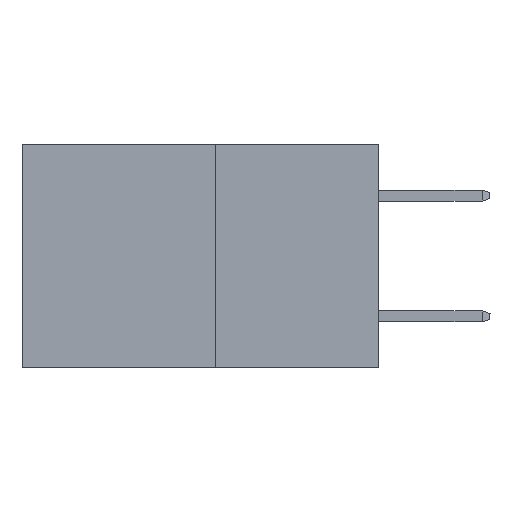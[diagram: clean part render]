
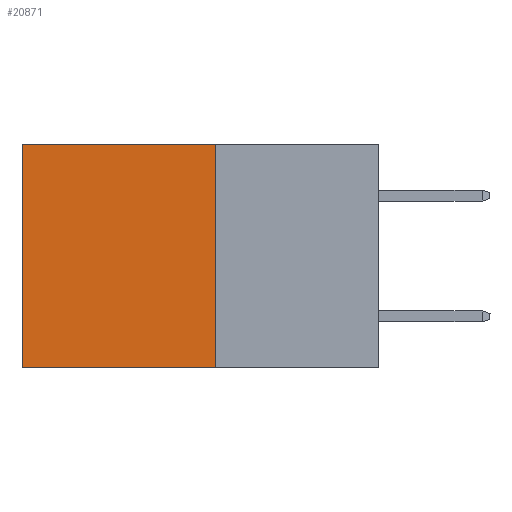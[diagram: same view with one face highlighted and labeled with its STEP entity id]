
A CAD part, left-side view. The second image highlights one B-rep face of the part: STEP entity #20871.
In plain terms, the highlighted planar face has unit normal (-1, 0, 0).
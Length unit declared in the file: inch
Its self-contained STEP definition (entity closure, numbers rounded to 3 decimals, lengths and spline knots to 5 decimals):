
#1173 = DIRECTION ( 'NONE',  ( 0., 0., -1. ) ) ;
#1309 = LINE ( 'NONE', #14296, #15281 ) ;
#1960 = EDGE_LOOP ( 'NONE', ( #15356, #31388, #6342, #3496 ) ) ;
#3225 = CARTESIAN_POINT ( 'NONE',  ( 0.277, 0.27, -0.37 ) ) ;
#3496 = ORIENTED_EDGE ( 'NONE', *, *, #25555, .T. ) ;
#3550 = LINE ( 'NONE', #9726, #30583 ) ;
#5328 = VECTOR ( 'NONE', #21414, 39.37008 ) ;
#6342 = ORIENTED_EDGE ( 'NONE', *, *, #32194, .F. ) ;
#6563 = EDGE_CURVE ( 'NONE', #22036, #18372, #15878, .T. ) ;
#7646 = DIRECTION ( 'NONE',  ( 0., 0., -1. ) ) ;
#8056 = VECTOR ( 'NONE', #33434, 39.37008 ) ;
#8473 = CARTESIAN_POINT ( 'NONE',  ( 0.277, 0.59, -0.37 ) ) ;
#9634 = CARTESIAN_POINT ( 'NONE',  ( 0.277, 0.59, 0. ) ) ;
#9726 = CARTESIAN_POINT ( 'NONE',  ( 0.277, 0.27, -0.37 ) ) ;
#10175 = CARTESIAN_POINT ( 'NONE',  ( 0.277, 0.27, -0.37 ) ) ;
#13587 = AXIS2_PLACEMENT_3D ( 'NONE', #10175, #23360, #7646 ) ;
#14296 = CARTESIAN_POINT ( 'NONE',  ( 0.277, 0.27, -0.37 ) ) ;
#15281 = VECTOR ( 'NONE', #1173, 39.37008 ) ;
#15356 = ORIENTED_EDGE ( 'NONE', *, *, #6563, .T. ) ;
#15665 = VERTEX_POINT ( 'NONE', #3225 ) ;
#15878 = LINE ( 'NONE', #30861, #8056 ) ;
#18372 = VERTEX_POINT ( 'NONE', #8473 ) ;
#18757 = CARTESIAN_POINT ( 'NONE',  ( 0.277, 0.27, 0. ) ) ;
#19546 = FACE_OUTER_BOUND ( 'NONE', #1960, .T. ) ;
#20094 = LINE ( 'NONE', #18757, #5328 ) ;
#20732 = EDGE_CURVE ( 'NONE', #15665, #18372, #3550, .T. ) ;
#20871 = ADVANCED_FACE ( 'NONE', ( #19546 ), #33678, .F. ) ;
#21414 = DIRECTION ( 'NONE',  ( 0., 1., 0. ) ) ;
#22036 = VERTEX_POINT ( 'NONE', #9634 ) ;
#22075 = CARTESIAN_POINT ( 'NONE',  ( 0.277, 0.27, 0. ) ) ;
#23360 = DIRECTION ( 'NONE',  ( 1., 0., 0. ) ) ;
#25424 = DIRECTION ( 'NONE',  ( 0., 1., 0. ) ) ;
#25555 = EDGE_CURVE ( 'NONE', #33575, #22036, #20094, .T. ) ;
#30583 = VECTOR ( 'NONE', #25424, 39.37008 ) ;
#30861 = CARTESIAN_POINT ( 'NONE',  ( 0.277, 0.59, -0.37 ) ) ;
#31388 = ORIENTED_EDGE ( 'NONE', *, *, #20732, .F. ) ;
#32194 = EDGE_CURVE ( 'NONE', #33575, #15665, #1309, .T. ) ;
#33434 = DIRECTION ( 'NONE',  ( 0., 0., -1. ) ) ;
#33575 = VERTEX_POINT ( 'NONE', #22075 ) ;
#33678 = PLANE ( 'NONE',  #13587 ) ;
